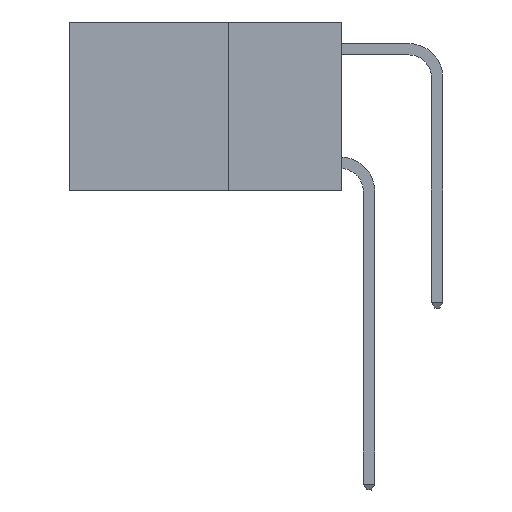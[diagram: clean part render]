
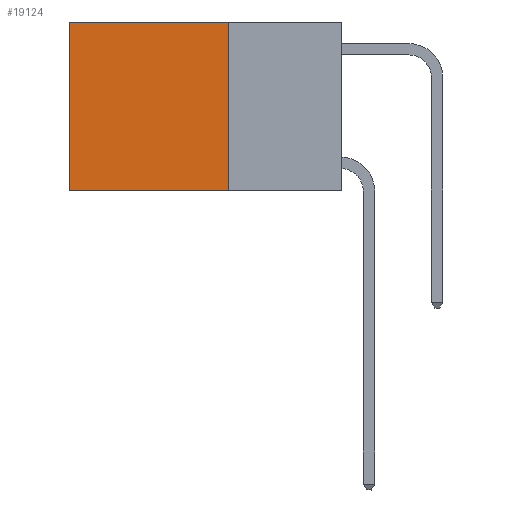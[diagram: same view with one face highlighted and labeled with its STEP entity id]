
A CAD part, left-side view. The second image highlights one B-rep face of the part: STEP entity #19124.
In plain terms, the highlighted planar face has unit normal (-1, 0, 0).
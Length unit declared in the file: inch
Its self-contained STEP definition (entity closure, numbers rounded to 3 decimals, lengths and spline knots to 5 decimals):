
#151 = LINE ( 'NONE', #6897, #8281 ) ;
#685 = ORIENTED_EDGE ( 'NONE', *, *, #8074, .T. ) ;
#1625 = EDGE_CURVE ( 'NONE', #5690, #19904, #151, .T. ) ;
#1648 = VERTEX_POINT ( 'NONE', #7167 ) ;
#1939 = EDGE_CURVE ( 'NONE', #9014, #5690, #4335, .T. ) ;
#2284 = CARTESIAN_POINT ( 'NONE',  ( 0.2625, 0.25, -0.37 ) ) ;
#3146 = LINE ( 'NONE', #14214, #15125 ) ;
#3501 = LINE ( 'NONE', #4604, #19598 ) ;
#3604 = DIRECTION ( 'NONE',  ( 0., 0., -1. ) ) ;
#4267 = DIRECTION ( 'NONE',  ( 0., 0., -1. ) ) ;
#4335 = LINE ( 'NONE', #8093, #7551 ) ;
#4604 = CARTESIAN_POINT ( 'NONE',  ( 0.2625, 0.25, 0. ) ) ;
#5690 = VERTEX_POINT ( 'NONE', #2284 ) ;
#6612 = FACE_OUTER_BOUND ( 'NONE', #16988, .T. ) ;
#6897 = CARTESIAN_POINT ( 'NONE',  ( 0.2625, 0.25, -0.37 ) ) ;
#7167 = CARTESIAN_POINT ( 'NONE',  ( 0.2625, 0.6, 0. ) ) ;
#7551 = VECTOR ( 'NONE', #3604, 39.37008 ) ;
#8074 = EDGE_CURVE ( 'NONE', #9014, #1648, #3501, .T. ) ;
#8093 = CARTESIAN_POINT ( 'NONE',  ( 0.2625, 0.25, 0. ) ) ;
#8281 = VECTOR ( 'NONE', #18003, 39.37008 ) ;
#8322 = ORIENTED_EDGE ( 'NONE', *, *, #1625, .F. ) ;
#8535 = ORIENTED_EDGE ( 'NONE', *, *, #10213, .T. ) ;
#8768 = ORIENTED_EDGE ( 'NONE', *, *, #1939, .F. ) ;
#9014 = VERTEX_POINT ( 'NONE', #15819 ) ;
#9609 = DIRECTION ( 'NONE',  ( 0., 0., -1. ) ) ;
#10213 = EDGE_CURVE ( 'NONE', #1648, #19904, #3146, .T. ) ;
#12092 = PLANE ( 'NONE',  #17003 ) ;
#13626 = DIRECTION ( 'NONE',  ( 1., 0., 0. ) ) ;
#14214 = CARTESIAN_POINT ( 'NONE',  ( 0.2625, 0.6, 0. ) ) ;
#15125 = VECTOR ( 'NONE', #9609, 39.37008 ) ;
#15819 = CARTESIAN_POINT ( 'NONE',  ( 0.2625, 0.25, 0. ) ) ;
#16988 = EDGE_LOOP ( 'NONE', ( #8535, #8322, #8768, #685 ) ) ;
#17003 = AXIS2_PLACEMENT_3D ( 'NONE', #18232, #13626, #4267 ) ;
#18003 = DIRECTION ( 'NONE',  ( 0., 1., 0. ) ) ;
#18232 = CARTESIAN_POINT ( 'NONE',  ( 0.2625, 0.25, 0. ) ) ;
#18586 = DIRECTION ( 'NONE',  ( 0., 1., 0. ) ) ;
#19124 = ADVANCED_FACE ( 'NONE', ( #6612 ), #12092, .F. ) ;
#19598 = VECTOR ( 'NONE', #18586, 39.37008 ) ;
#19904 = VERTEX_POINT ( 'NONE', #20212 ) ;
#20212 = CARTESIAN_POINT ( 'NONE',  ( 0.2625, 0.6, -0.37 ) ) ;
